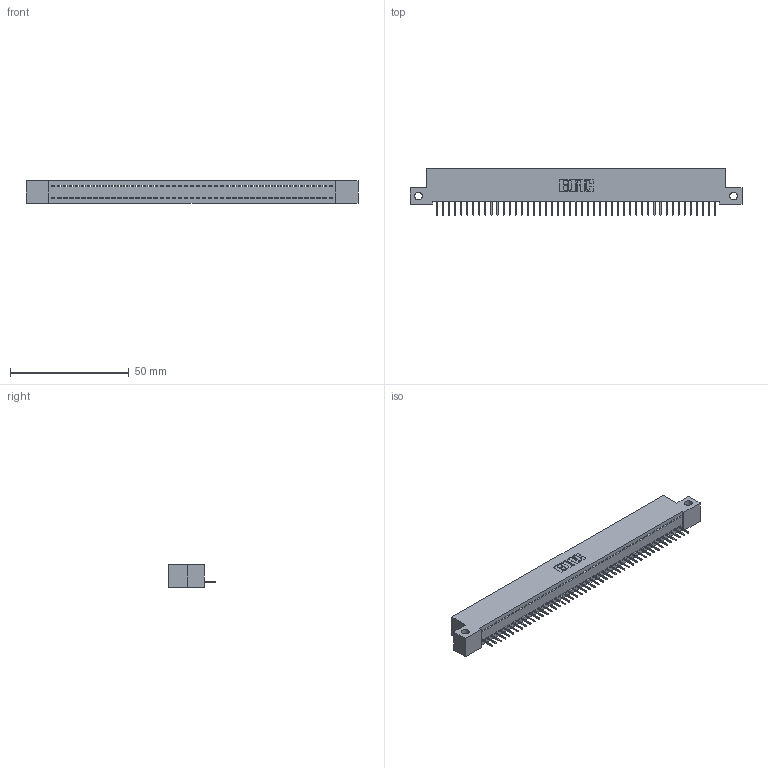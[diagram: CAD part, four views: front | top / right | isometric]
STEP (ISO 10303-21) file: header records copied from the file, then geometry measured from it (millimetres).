
FILE_DESCRIPTION (( 'STEP AP203' ), '1' );
FILE_NAME ('342-047-524-112.STEP', '2019-10-02T21:18:14', ( '' ), ( '' ), 'SwSTEP 2.0', 'SolidWorks 2016', '' );
FILE_SCHEMA (( 'CONFIG_CONTROL_DESIGN' ));
Length unit declared in the file: inch
Products named in the file (3): 342 Part_Side Mount; 345-292-001_345-293-124; 342-047-524-112
Assembly tree (48 placements, depth 2):
  342-047-524-112
    342 Part_Side Mount
    345-292-001_345-293-124  x47
Bounding box: 139.7 x 19.69 x 9.4 mm (x, y, z)
Volume: 12007.7 mm3; surface area: 16986.4 mm2
Topology: 48 solids, 48 shells, 3024 faces, 8759 edges, 5650 vertices
Faces by surface type: plane 2322, cylinder 702
Entity records: 28031 total; most frequent: CARTESIAN_POINT 4839, ORIENTED_EDGE 4822, DIRECTION 4073, EDGE_CURVE 2411, VECTOR 2287, LINE 2287, VERTEX_POINT 1602, AXIS2_PLACEMENT_3D 893
